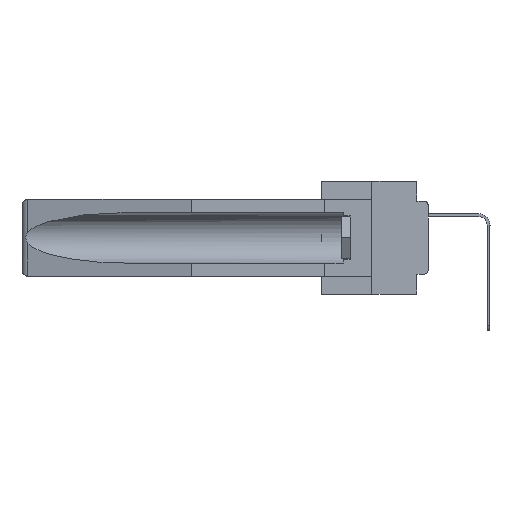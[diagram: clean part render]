
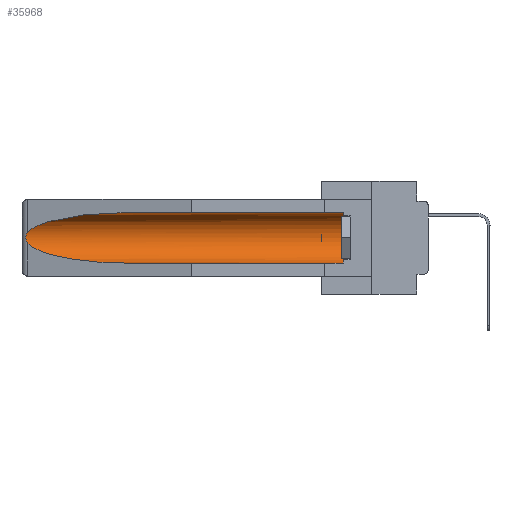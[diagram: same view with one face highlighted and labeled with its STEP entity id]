
A CAD part, left-side view. The second image highlights one B-rep face of the part: STEP entity #35968.
In plain terms, the highlighted cylindrical face has radius 2.857 mm (diameter 5.715 mm), a partial arc.
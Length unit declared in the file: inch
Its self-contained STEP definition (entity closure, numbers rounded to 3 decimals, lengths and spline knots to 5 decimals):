
#287 = DIRECTION ( 'NONE',  ( 0., 1., 0. ) ) ;
#503 = LINE ( 'NONE', #34510, #25135 ) ;
#557 = DIRECTION ( 'NONE',  ( 0., 0., 1. ) ) ;
#1001 = AXIS2_PLACEMENT_3D ( 'NONE', #37861, #13813, #32563 ) ;
#1453 = EDGE_LOOP ( 'NONE', ( #7104, #27284, #30525, #37799, #9167, #28410 ) ) ;
#3749 = CARTESIAN_POINT ( 'NONE',  ( 0.2673, 1.53269, -0.17917 ) ) ;
#4297 = CARTESIAN_POINT ( 'NONE',  ( 0.155, 0.126, -0.059 ) ) ;
#6387 = CARTESIAN_POINT ( 'NONE',  ( 0.2675, 1.53308, -0.16763 ) ) ;
#7090 = VERTEX_POINT ( 'NONE', #31911 ) ;
#7104 = ORIENTED_EDGE ( 'NONE', *, *, #34042, .T. ) ;
#7769 = CARTESIAN_POINT ( 'NONE',  ( 0.26537, 1.52718, -0.19328 ) ) ;
#7920 = EDGE_CURVE ( 'NONE', #19638, #17739, #20377, .T. ) ;
#8733 = LINE ( 'NONE', #35089, #22758 ) ;
#9128 = EDGE_CURVE ( 'NONE', #7090, #33865, #28699, .T. ) ;
#9167 = ORIENTED_EDGE ( 'NONE', *, *, #9128, .T. ) ;
#9448 =( BOUNDED_CURVE ( )  B_SPLINE_CURVE ( 3, ( #26566, #29690, #26432, #23041 ),
 .UNSPECIFIED., .F., .F. ) 
 B_SPLINE_CURVE_WITH_KNOTS ( ( 4, 4 ),
 ( 4.71239, 6.08839 ),
 .UNSPECIFIED. ) 
 CURVE ( )  GEOMETRIC_REPRESENTATION_ITEM ( )  RATIONAL_B_SPLINE_CURVE ( ( 1., 0.848, 0.848, 1. ) ) 
 REPRESENTATION_ITEM ( '' )  );
#9638 = CARTESIAN_POINT ( 'NONE',  ( 0.26655, 1.53094, -0.18657 ) ) ;
#11264 = EDGE_CURVE ( 'NONE', #32495, #19638, #31759, .T. ) ;
#12800 = CARTESIAN_POINT ( 'NONE',  ( 0.26537, 1.52718, -0.14972 ) ) ;
#13680 = CARTESIAN_POINT ( 'NONE',  ( 0.26537, 1.52718, -0.14972 ) ) ;
#13813 = DIRECTION ( 'NONE',  ( 0., -1., 0. ) ) ;
#14319 = CARTESIAN_POINT ( 'NONE',  ( 0.21114, 1.30732, -0.284 ) ) ;
#15643 = CARTESIAN_POINT ( 'NONE',  ( 0.26597, 1.52961, -0.15275 ) ) ;
#15926 = CARTESIAN_POINT ( 'NONE',  ( 0.26654, 1.53092, -0.15636 ) ) ;
#16056 = CARTESIAN_POINT ( 'NONE',  ( 0.2673, 1.5327, -0.16383 ) ) ;
#17739 = VERTEX_POINT ( 'NONE', #35637 ) ;
#19638 = VERTEX_POINT ( 'NONE', #39973 ) ;
#20377 =( BOUNDED_CURVE ( )  B_SPLINE_CURVE ( 3, ( #7769, #39011, #14319, #32804 ),
 .UNSPECIFIED., .F., .F. ) 
 B_SPLINE_CURVE_WITH_KNOTS ( ( 4, 4 ),
 ( 0.1948, 1.5708 ),
 .UNSPECIFIED. ) 
 CURVE ( )  GEOMETRIC_REPRESENTATION_ITEM ( )  RATIONAL_B_SPLINE_CURVE ( ( 1., 0.848, 0.848, 1. ) ) 
 REPRESENTATION_ITEM ( '' )  );
#20525 = EDGE_CURVE ( 'NONE', #33865, #28314, #503, .T. ) ;
#22217 = CARTESIAN_POINT ( 'NONE',  ( 0.2675, 1.53308, -0.17534 ) ) ;
#22758 = VECTOR ( 'NONE', #29025, 39.37008 ) ;
#23041 = CARTESIAN_POINT ( 'NONE',  ( 0.26537, 1.52718, -0.14972 ) ) ;
#25135 = VECTOR ( 'NONE', #28297, 39.37008 ) ;
#26432 = CARTESIAN_POINT ( 'NONE',  ( 0.25451, 1.48313, -0.09465 ) ) ;
#26566 = CARTESIAN_POINT ( 'NONE',  ( 0.155, 1.07973, -0.059 ) ) ;
#27272 = AXIS2_PLACEMENT_3D ( 'NONE', #37306, #287, #557 ) ;
#27284 = ORIENTED_EDGE ( 'NONE', *, *, #11264, .T. ) ;
#27737 = CARTESIAN_POINT ( 'NONE',  ( 0.155, 1.07973, -0.059 ) ) ;
#28297 = DIRECTION ( 'NONE',  ( 0., 1., 0. ) ) ;
#28314 = VERTEX_POINT ( 'NONE', #27737 ) ;
#28410 = ORIENTED_EDGE ( 'NONE', *, *, #20525, .T. ) ;
#28699 = CIRCLE ( 'NONE', #1001, 0.1125 ) ;
#29025 = DIRECTION ( 'NONE',  ( 0., 1., 0. ) ) ;
#29458 = CYLINDRICAL_SURFACE ( 'NONE', #27272, 0.1125 ) ;
#29690 = CARTESIAN_POINT ( 'NONE',  ( 0.21114, 1.30732, -0.059 ) ) ;
#29931 = FACE_OUTER_BOUND ( 'NONE', #1453, .T. ) ;
#30525 = ORIENTED_EDGE ( 'NONE', *, *, #7920, .T. ) ;
#31759 = B_SPLINE_CURVE_WITH_KNOTS ( 'NONE', 3,
 ( #12800, #15643, #15926, #16056, #6387, #22217, #3749, #9638, #34385, #37495 ),
 .UNSPECIFIED., .F., .F.,
 ( 4, 2, 2, 2, 4 ),
 ( 0., 0.00029, 0.00058, 0.00087, 0.00117 ),
 .UNSPECIFIED. ) ;
#31911 = CARTESIAN_POINT ( 'NONE',  ( 0.155, 0.126, -0.284 ) ) ;
#32495 = VERTEX_POINT ( 'NONE', #13680 ) ;
#32563 = DIRECTION ( 'NONE',  ( 0., 0., 1. ) ) ;
#32804 = CARTESIAN_POINT ( 'NONE',  ( 0.155, 1.07973, -0.284 ) ) ;
#33865 = VERTEX_POINT ( 'NONE', #4297 ) ;
#34042 = EDGE_CURVE ( 'NONE', #28314, #32495, #9448, .T. ) ;
#34385 = CARTESIAN_POINT ( 'NONE',  ( 0.26597, 1.5296, -0.19026 ) ) ;
#34510 = CARTESIAN_POINT ( 'NONE',  ( 0.155, -0.30754, -0.059 ) ) ;
#35089 = CARTESIAN_POINT ( 'NONE',  ( 0.155, -0.30754, -0.284 ) ) ;
#35637 = CARTESIAN_POINT ( 'NONE',  ( 0.155, 1.07973, -0.284 ) ) ;
#35968 = ADVANCED_FACE ( 'NONE', ( #29931 ), #29458, .F. ) ;
#36848 = EDGE_CURVE ( 'NONE', #7090, #17739, #8733, .T. ) ;
#37306 = CARTESIAN_POINT ( 'NONE',  ( 0.155, -0.30754, -0.1715 ) ) ;
#37495 = CARTESIAN_POINT ( 'NONE',  ( 0.26537, 1.52718, -0.19328 ) ) ;
#37799 = ORIENTED_EDGE ( 'NONE', *, *, #36848, .F. ) ;
#37861 = CARTESIAN_POINT ( 'NONE',  ( 0.155, 0.126, -0.1715 ) ) ;
#39011 = CARTESIAN_POINT ( 'NONE',  ( 0.25451, 1.48313, -0.24835 ) ) ;
#39973 = CARTESIAN_POINT ( 'NONE',  ( 0.26537, 1.52718, -0.19328 ) ) ;
